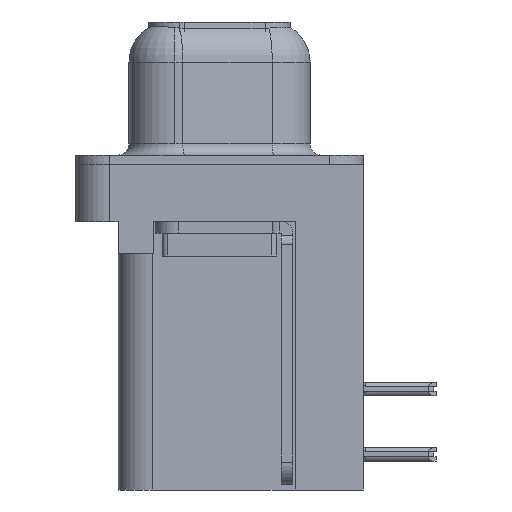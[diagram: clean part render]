
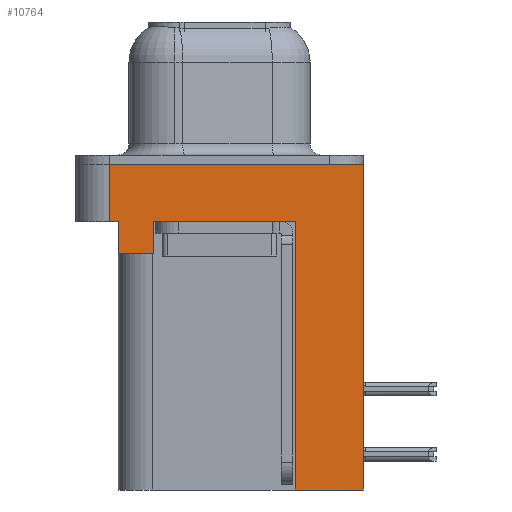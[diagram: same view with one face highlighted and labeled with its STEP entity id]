
A CAD part, left-side view. The second image highlights one B-rep face of the part: STEP entity #10764.
In plain terms, the highlighted planar face has unit normal (-1, 0, 0).
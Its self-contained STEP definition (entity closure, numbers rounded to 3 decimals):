
#667 = EDGE_CURVE ( 'NONE', #9177, #11331, #2251, .T. ) ;
#1043 = ORIENTED_EDGE ( 'NONE', *, *, #667, .T. ) ;
#1102 = CARTESIAN_POINT ( 'NONE',  ( -3., 2.895, -3.9 ) ) ;
#1277 = ORIENTED_EDGE ( 'NONE', *, *, #28880, .F. ) ;
#1396 = DIRECTION ( 'NONE',  ( 0., -1., 0. ) ) ;
#1474 = ORIENTED_EDGE ( 'NONE', *, *, #12364, .T. ) ;
#2251 = LINE ( 'NONE', #21369, #6469 ) ;
#3619 = VECTOR ( 'NONE', #15804, 1000. ) ;
#3901 = VERTEX_POINT ( 'NONE', #1102 ) ;
#4268 = LINE ( 'NONE', #25736, #10884 ) ;
#4628 = CARTESIAN_POINT ( 'NONE',  ( -3., 4.775, -2.5 ) ) ;
#4796 = EDGE_CURVE ( 'NONE', #28165, #11331, #5945, .T. ) ;
#4984 = DIRECTION ( 'NONE',  ( 0., 1., 0. ) ) ;
#5778 = DIRECTION ( 'NONE',  ( 0., -1., 0. ) ) ;
#5945 = LINE ( 'NONE', #27741, #13045 ) ;
#5980 = CARTESIAN_POINT ( 'NONE',  ( -3., -3.295, -2.5 ) ) ;
#6469 = VECTOR ( 'NONE', #8818, 1000. ) ;
#6604 = DIRECTION ( 'NONE',  ( 0., 1., 0. ) ) ;
#8001 = ORIENTED_EDGE ( 'NONE', *, *, #25871, .F. ) ;
#8350 = EDGE_CURVE ( 'NONE', #14370, #24024, #29934, .T. ) ;
#8397 = ORIENTED_EDGE ( 'NONE', *, *, #12717, .F. ) ;
#8698 = AXIS2_PLACEMENT_3D ( 'NONE', #25561, #11137, #20553 ) ;
#8818 = DIRECTION ( 'NONE',  ( 0., 0., 1. ) ) ;
#8898 = CARTESIAN_POINT ( 'NONE',  ( -3., -6.275, 0. ) ) ;
#9177 = VERTEX_POINT ( 'NONE', #24378 ) ;
#9197 = LINE ( 'NONE', #12023, #9800 ) ;
#9539 = DIRECTION ( 'NONE',  ( 0., 0., 1. ) ) ;
#9800 = VECTOR ( 'NONE', #4984, 1000. ) ;
#9913 = ORIENTED_EDGE ( 'NONE', *, *, #11678, .T. ) ;
#10234 = VECTOR ( 'NONE', #17056, 1000. ) ;
#10764 = ADVANCED_FACE ( 'NONE', ( #16006 ), #13494, .T. ) ;
#10884 = VECTOR ( 'NONE', #6604, 1000. ) ;
#11137 = DIRECTION ( 'NONE',  ( -1., 0., 0. ) ) ;
#11331 = VERTEX_POINT ( 'NONE', #8898 ) ;
#11567 = EDGE_CURVE ( 'NONE', #28789, #24024, #12954, .T. ) ;
#11678 = EDGE_CURVE ( 'NONE', #3901, #19284, #25174, .T. ) ;
#11945 = ORIENTED_EDGE ( 'NONE', *, *, #26929, .F. ) ;
#11969 = CARTESIAN_POINT ( 'NONE',  ( -3., 2.895, -2.5 ) ) ;
#12023 = CARTESIAN_POINT ( 'NONE',  ( -3., -3.295, -14.2 ) ) ;
#12364 = EDGE_CURVE ( 'NONE', #19284, #29050, #29169, .T. ) ;
#12717 = EDGE_CURVE ( 'NONE', #9177, #19708, #9197, .T. ) ;
#12954 = LINE ( 'NONE', #22522, #10234 ) ;
#13045 = VECTOR ( 'NONE', #1396, 1000. ) ;
#13412 = ORIENTED_EDGE ( 'NONE', *, *, #4796, .F. ) ;
#13494 = PLANE ( 'NONE',  #8698 ) ;
#13568 = CARTESIAN_POINT ( 'NONE',  ( -3., 2.895, -3.9 ) ) ;
#14370 = VERTEX_POINT ( 'NONE', #27692 ) ;
#14881 = LINE ( 'NONE', #26651, #18787 ) ;
#14921 = CARTESIAN_POINT ( 'NONE',  ( -3., 4.775, 0. ) ) ;
#15344 = CARTESIAN_POINT ( 'NONE',  ( -3., 4.425, -3.9 ) ) ;
#15804 = DIRECTION ( 'NONE',  ( 0., 0., 1. ) ) ;
#16006 = FACE_OUTER_BOUND ( 'NONE', #25667, .T. ) ;
#17056 = DIRECTION ( 'NONE',  ( 0., -1., 0. ) ) ;
#18343 = VECTOR ( 'NONE', #9539, 1000. ) ;
#18787 = VECTOR ( 'NONE', #21619, 1000. ) ;
#19284 = VERTEX_POINT ( 'NONE', #11969 ) ;
#19708 = VERTEX_POINT ( 'NONE', #22414 ) ;
#20553 = DIRECTION ( 'NONE',  ( 0., 0., 1. ) ) ;
#21272 = VECTOR ( 'NONE', #27851, 1000. ) ;
#21369 = CARTESIAN_POINT ( 'NONE',  ( -3., -6.275, -2.5 ) ) ;
#21619 = DIRECTION ( 'NONE',  ( 0., 0., 1. ) ) ;
#22414 = CARTESIAN_POINT ( 'NONE',  ( -3., -3.295, -14.2 ) ) ;
#22522 = CARTESIAN_POINT ( 'NONE',  ( -3., -6.275, -2.5 ) ) ;
#23475 = ORIENTED_EDGE ( 'NONE', *, *, #11567, .T. ) ;
#23654 = CARTESIAN_POINT ( 'NONE',  ( -3., 4.425, -2.5 ) ) ;
#23792 = VECTOR ( 'NONE', #5778, 1000. ) ;
#23977 = LINE ( 'NONE', #28862, #18343 ) ;
#24024 = VERTEX_POINT ( 'NONE', #23654 ) ;
#24378 = CARTESIAN_POINT ( 'NONE',  ( -3., -6.275, -14.2 ) ) ;
#24569 = ORIENTED_EDGE ( 'NONE', *, *, #8350, .F. ) ;
#25174 = LINE ( 'NONE', #13568, #21272 ) ;
#25561 = CARTESIAN_POINT ( 'NONE',  ( -3., -6.275, -2.5 ) ) ;
#25667 = EDGE_LOOP ( 'NONE', ( #13412, #8001, #23475, #24569, #1277, #9913, #1474, #11945, #8397, #1043 ) ) ;
#25736 = CARTESIAN_POINT ( 'NONE',  ( -3., 4.425, -3.9 ) ) ;
#25871 = EDGE_CURVE ( 'NONE', #28789, #28165, #14881, .T. ) ;
#26651 = CARTESIAN_POINT ( 'NONE',  ( -3., 4.775, -2.5 ) ) ;
#26929 = EDGE_CURVE ( 'NONE', #19708, #29050, #23977, .T. ) ;
#26972 = CARTESIAN_POINT ( 'NONE',  ( -3., -6.275, -2.5 ) ) ;
#27692 = CARTESIAN_POINT ( 'NONE',  ( -3., 4.425, -3.9 ) ) ;
#27741 = CARTESIAN_POINT ( 'NONE',  ( -3., -6.275, 0. ) ) ;
#27851 = DIRECTION ( 'NONE',  ( 0., 0., 1. ) ) ;
#28165 = VERTEX_POINT ( 'NONE', #14921 ) ;
#28789 = VERTEX_POINT ( 'NONE', #4628 ) ;
#28862 = CARTESIAN_POINT ( 'NONE',  ( -3., -3.295, -14.2 ) ) ;
#28880 = EDGE_CURVE ( 'NONE', #3901, #14370, #4268, .T. ) ;
#29050 = VERTEX_POINT ( 'NONE', #5980 ) ;
#29169 = LINE ( 'NONE', #26972, #23792 ) ;
#29934 = LINE ( 'NONE', #15344, #3619 ) ;
